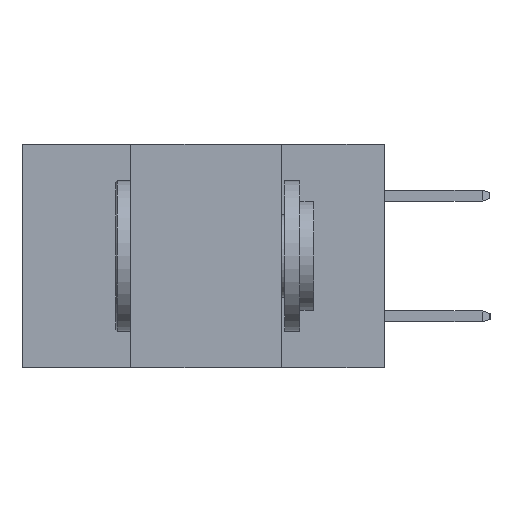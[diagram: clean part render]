
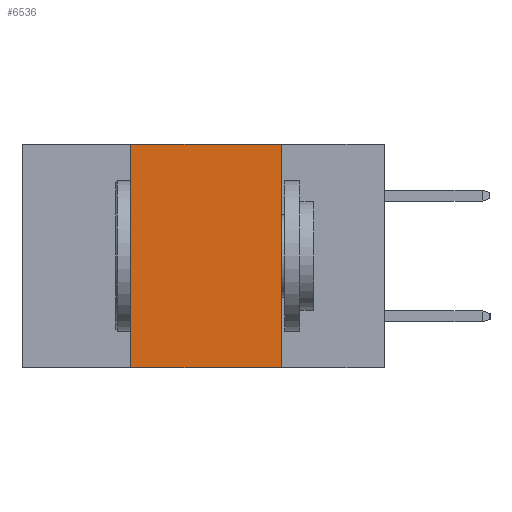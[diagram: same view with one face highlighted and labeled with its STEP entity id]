
A CAD part, left-side view. The second image highlights one B-rep face of the part: STEP entity #6536.
In plain terms, the highlighted planar face has unit normal (-1, 0, 0).
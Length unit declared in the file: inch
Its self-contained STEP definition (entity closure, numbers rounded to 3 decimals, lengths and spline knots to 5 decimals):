
#6 = ORIENTED_EDGE ( 'NONE', *, *, #7577, .F. ) ;
#236 = ORIENTED_EDGE ( 'NONE', *, *, #10418, .F. ) ;
#604 = CARTESIAN_POINT ( 'NONE',  ( 0., 0.42, 0. ) ) ;
#774 = VERTEX_POINT ( 'NONE', #9018 ) ;
#1183 = LINE ( 'NONE', #2036, #5797 ) ;
#1522 = VERTEX_POINT ( 'NONE', #6396 ) ;
#2036 = CARTESIAN_POINT ( 'NONE',  ( 0., 0.17, -0.37 ) ) ;
#3130 = ORIENTED_EDGE ( 'NONE', *, *, #3321, .T. ) ;
#3321 = EDGE_CURVE ( 'NONE', #774, #1522, #10196, .T. ) ;
#3439 = DIRECTION ( 'NONE',  ( 0., -1., 0. ) ) ;
#3860 = DIRECTION ( 'NONE',  ( 1., 0., 0. ) ) ;
#3905 = VECTOR ( 'NONE', #3439, 39.37008 ) ;
#4156 = VECTOR ( 'NONE', #4774, 39.37008 ) ;
#4202 = LINE ( 'NONE', #5245, #3905 ) ;
#4429 = LINE ( 'NONE', #10827, #4156 ) ;
#4774 = DIRECTION ( 'NONE',  ( 0., 0., 1. ) ) ;
#5050 = ORIENTED_EDGE ( 'NONE', *, *, #9289, .F. ) ;
#5245 = CARTESIAN_POINT ( 'NONE',  ( 0., 0.6, 0. ) ) ;
#5326 = FACE_OUTER_BOUND ( 'NONE', #10021, .T. ) ;
#5338 = VECTOR ( 'NONE', #10805, 39.37008 ) ;
#5619 = CARTESIAN_POINT ( 'NONE',  ( 0., 0.6, 0. ) ) ;
#5797 = VECTOR ( 'NONE', #10806, 39.37008 ) ;
#6396 = CARTESIAN_POINT ( 'NONE',  ( 0., 0.17, -0.37 ) ) ;
#6536 = ADVANCED_FACE ( 'NONE', ( #5326 ), #9078, .F. ) ;
#7577 = EDGE_CURVE ( 'NONE', #9471, #7607, #4202, .T. ) ;
#7607 = VERTEX_POINT ( 'NONE', #10437 ) ;
#7808 = AXIS2_PLACEMENT_3D ( 'NONE', #5619, #3860, #9937 ) ;
#9018 = CARTESIAN_POINT ( 'NONE',  ( 0., 0.42, -0.37 ) ) ;
#9078 = PLANE ( 'NONE',  #7808 ) ;
#9289 = EDGE_CURVE ( 'NONE', #774, #9471, #4429, .T. ) ;
#9471 = VERTEX_POINT ( 'NONE', #604 ) ;
#9937 = DIRECTION ( 'NONE',  ( 0., 0., -1. ) ) ;
#10021 = EDGE_LOOP ( 'NONE', ( #236, #6, #5050, #3130 ) ) ;
#10196 = LINE ( 'NONE', #10792, #5338 ) ;
#10418 = EDGE_CURVE ( 'NONE', #7607, #1522, #1183, .T. ) ;
#10437 = CARTESIAN_POINT ( 'NONE',  ( 0., 0.17, 0. ) ) ;
#10792 = CARTESIAN_POINT ( 'NONE',  ( 0., 0.6, -0.37 ) ) ;
#10805 = DIRECTION ( 'NONE',  ( 0., -1., 0. ) ) ;
#10806 = DIRECTION ( 'NONE',  ( 0., 0., -1. ) ) ;
#10827 = CARTESIAN_POINT ( 'NONE',  ( 0., 0.42, -0.37 ) ) ;
